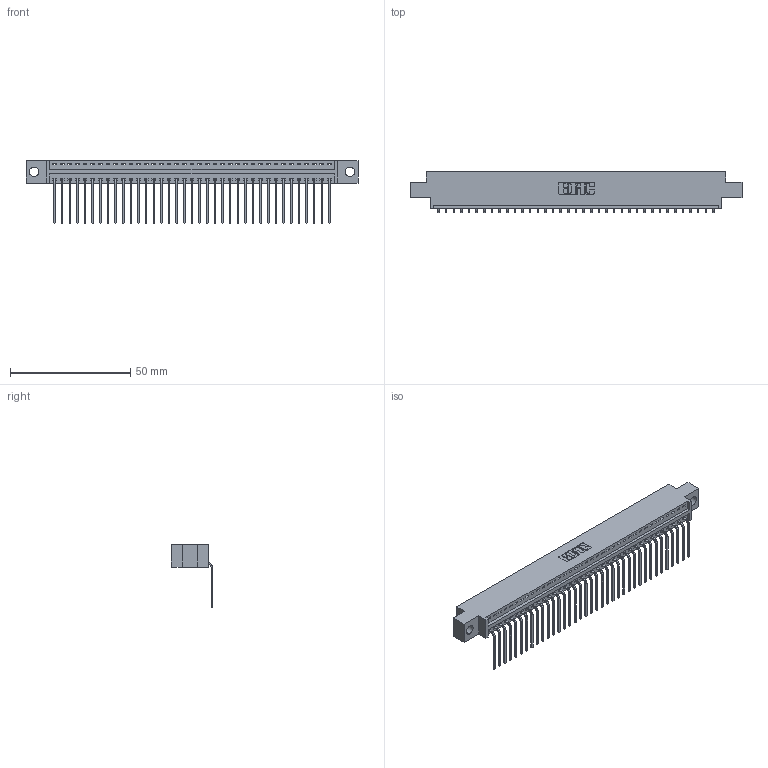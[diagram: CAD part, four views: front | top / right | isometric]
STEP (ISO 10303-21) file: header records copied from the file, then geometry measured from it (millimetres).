
FILE_DESCRIPTION (( 'STEP AP203' ), '1' );
FILE_NAME ('396-037-559-604.STEP', '2019-10-31T22:29:20', ( '' ), ( '' ), 'SwSTEP 2.0', 'SolidWorks 2016', '' );
FILE_SCHEMA (( 'CONFIG_CONTROL_DESIGN' ));
Length unit declared in the file: inch
Products named in the file (3): 346 Part_0.170 Offset - 0.156 Dia-TH; 345-292-001_558 559 Tail - 1; 396-037-559-604
Assembly tree (38 placements, depth 2):
  396-037-559-604
    346 Part_0.170 Offset - 0.156 Dia-TH
    345-292-001_558 559 Tail - 1  x37
Bounding box: 138.05 x 17.08 x 26.16 mm (x, y, z)
Volume: 13060.7 mm3; surface area: 16971 mm2
Topology: 38 solids, 38 shells, 2346 faces, 7075 edges, 4666 vertices
Faces by surface type: plane 1634, cylinder 712
Entity records: 23855 total; most frequent: CARTESIAN_POINT 4099, ORIENTED_EDGE 4070, DIRECTION 3621, EDGE_CURVE 2035, LINE 1755, VECTOR 1755, VERTEX_POINT 1354, AXIS2_PLACEMENT_3D 933
